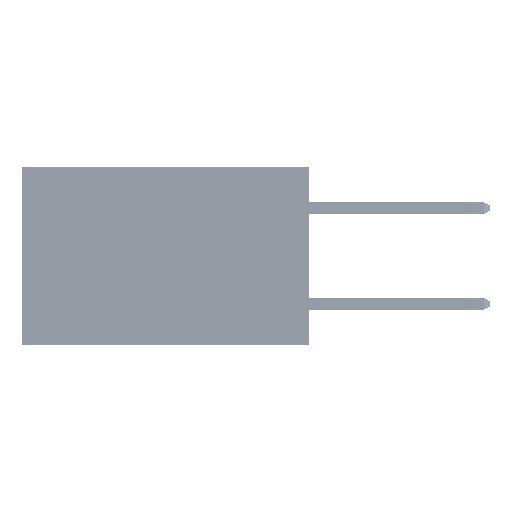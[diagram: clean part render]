
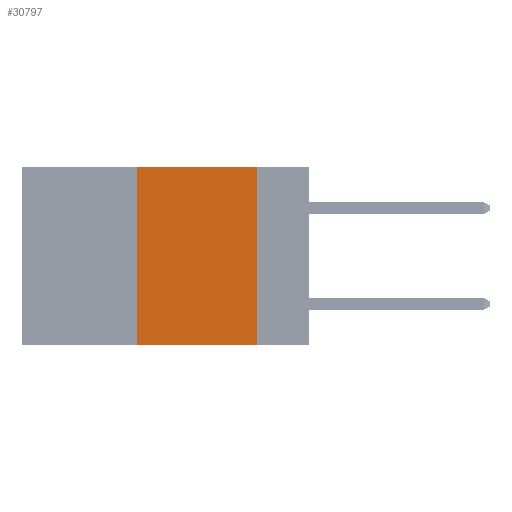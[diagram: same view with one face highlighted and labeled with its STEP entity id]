
A CAD part, left-side view. The second image highlights one B-rep face of the part: STEP entity #30797.
In plain terms, the highlighted planar face has unit normal (-1, 0, 0).
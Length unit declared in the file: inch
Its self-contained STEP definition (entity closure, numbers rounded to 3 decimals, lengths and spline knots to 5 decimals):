
#817 = CARTESIAN_POINT ( 'NONE',  ( 0., 0.11, -0.37 ) ) ;
#1767 = LINE ( 'NONE', #10034, #49146 ) ;
#3292 = CARTESIAN_POINT ( 'NONE',  ( 0., 0.36, -0.37 ) ) ;
#4078 = VERTEX_POINT ( 'NONE', #3292 ) ;
#4162 = VECTOR ( 'NONE', #41167, 39.37008 ) ;
#7942 = VECTOR ( 'NONE', #18394, 39.37008 ) ;
#9540 = EDGE_CURVE ( 'NONE', #4078, #41364, #1767, .T. ) ;
#9691 = DIRECTION ( 'NONE',  ( 1., 0., 0. ) ) ;
#10034 = CARTESIAN_POINT ( 'NONE',  ( 0., 0.36, 0. ) ) ;
#13728 = DIRECTION ( 'NONE',  ( 0., -1., 0. ) ) ;
#13868 = VECTOR ( 'NONE', #13728, 39.37008 ) ;
#17141 = ORIENTED_EDGE ( 'NONE', *, *, #27364, .F. ) ;
#18203 = CARTESIAN_POINT ( 'NONE',  ( 0., 0.6, 0. ) ) ;
#18358 = LINE ( 'NONE', #26127, #4162 ) ;
#18394 = DIRECTION ( 'NONE',  ( 0., 0., -1. ) ) ;
#18481 = VERTEX_POINT ( 'NONE', #817 ) ;
#22103 = PLANE ( 'NONE',  #32342 ) ;
#22358 = DIRECTION ( 'NONE',  ( 0., 0., -1. ) ) ;
#24368 = ORIENTED_EDGE ( 'NONE', *, *, #42813, .F. ) ;
#26127 = CARTESIAN_POINT ( 'NONE',  ( 0., 0.6, 0. ) ) ;
#27226 = EDGE_LOOP ( 'NONE', ( #24368, #17141, #44120, #28179 ) ) ;
#27364 = EDGE_CURVE ( 'NONE', #41364, #38293, #18358, .T. ) ;
#27466 = CARTESIAN_POINT ( 'NONE',  ( 0., 0.11, 0. ) ) ;
#28179 = ORIENTED_EDGE ( 'NONE', *, *, #45234, .T. ) ;
#30797 = ADVANCED_FACE ( 'NONE', ( #38142 ), #22103, .F. ) ;
#31083 = LINE ( 'NONE', #27466, #7942 ) ;
#32342 = AXIS2_PLACEMENT_3D ( 'NONE', #18203, #9691, #22358 ) ;
#33387 = LINE ( 'NONE', #49179, #13868 ) ;
#34118 = CARTESIAN_POINT ( 'NONE',  ( 0., 0.36, 0. ) ) ;
#38142 = FACE_OUTER_BOUND ( 'NONE', #27226, .T. ) ;
#38293 = VERTEX_POINT ( 'NONE', #48182 ) ;
#41167 = DIRECTION ( 'NONE',  ( 0., -1., 0. ) ) ;
#41364 = VERTEX_POINT ( 'NONE', #34118 ) ;
#42813 = EDGE_CURVE ( 'NONE', #38293, #18481, #31083, .T. ) ;
#44120 = ORIENTED_EDGE ( 'NONE', *, *, #9540, .F. ) ;
#45234 = EDGE_CURVE ( 'NONE', #4078, #18481, #33387, .T. ) ;
#45735 = DIRECTION ( 'NONE',  ( 0., 0., 1. ) ) ;
#48182 = CARTESIAN_POINT ( 'NONE',  ( 0., 0.11, 0. ) ) ;
#49146 = VECTOR ( 'NONE', #45735, 39.37008 ) ;
#49179 = CARTESIAN_POINT ( 'NONE',  ( 0., 0.6, -0.37 ) ) ;
